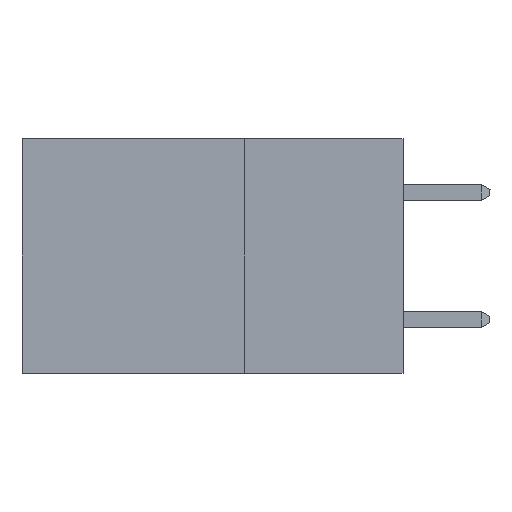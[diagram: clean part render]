
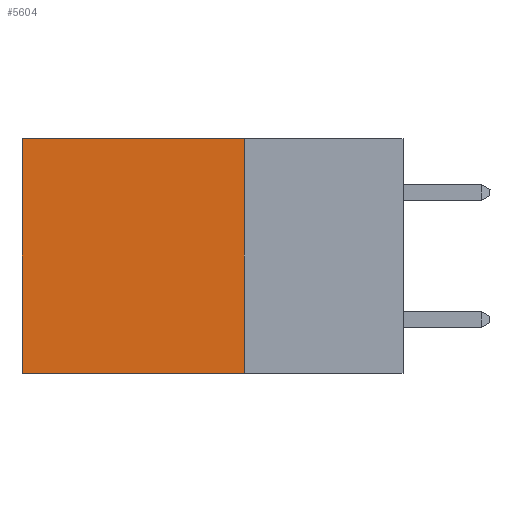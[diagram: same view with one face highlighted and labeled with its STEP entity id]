
A CAD part, left-side view. The second image highlights one B-rep face of the part: STEP entity #5604.
In plain terms, the highlighted planar face has unit normal (-1, 0, 0).
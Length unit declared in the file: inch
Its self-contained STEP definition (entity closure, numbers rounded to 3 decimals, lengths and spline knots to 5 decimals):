
#353 = DIRECTION ( 'NONE',  ( 0., 0., -1. ) ) ;
#376 = CARTESIAN_POINT ( 'NONE',  ( 0.2875, 0.6, 0. ) ) ;
#476 = ORIENTED_EDGE ( 'NONE', *, *, #1804, .F. ) ;
#590 = DIRECTION ( 'NONE',  ( 0., 1., 0. ) ) ;
#1067 = EDGE_CURVE ( 'NONE', #9309, #5365, #3315, .T. ) ;
#1146 = CARTESIAN_POINT ( 'NONE',  ( 0.2875, 0.6, -0.37 ) ) ;
#1309 = ORIENTED_EDGE ( 'NONE', *, *, #3666, .F. ) ;
#1804 = EDGE_CURVE ( 'NONE', #9309, #7388, #7428, .T. ) ;
#2971 = VECTOR ( 'NONE', #5877, 39.37008 ) ;
#3315 = LINE ( 'NONE', #4291, #5368 ) ;
#3666 = EDGE_CURVE ( 'NONE', #7388, #3703, #10018, .T. ) ;
#3703 = VERTEX_POINT ( 'NONE', #1146 ) ;
#3717 = EDGE_CURVE ( 'NONE', #5365, #3703, #4565, .T. ) ;
#3999 = CARTESIAN_POINT ( 'NONE',  ( 0.2875, 0.25, 0. ) ) ;
#4291 = CARTESIAN_POINT ( 'NONE',  ( 0.2875, 0.25, 0. ) ) ;
#4565 = LINE ( 'NONE', #10468, #2971 ) ;
#5197 = CARTESIAN_POINT ( 'NONE',  ( 0.2875, 0.25, -0.37 ) ) ;
#5365 = VERTEX_POINT ( 'NONE', #376 ) ;
#5368 = VECTOR ( 'NONE', #590, 39.37008 ) ;
#5604 = ADVANCED_FACE ( 'NONE', ( #7890 ), #9031, .F. ) ;
#5877 = DIRECTION ( 'NONE',  ( 0., 0., -1. ) ) ;
#6219 = VECTOR ( 'NONE', #11779, 39.37008 ) ;
#6261 = CARTESIAN_POINT ( 'NONE',  ( 0.2875, 0.25, 0. ) ) ;
#6306 = CARTESIAN_POINT ( 'NONE',  ( 0.2875, 0.25, 0. ) ) ;
#7107 = AXIS2_PLACEMENT_3D ( 'NONE', #6306, #10928, #7285 ) ;
#7285 = DIRECTION ( 'NONE',  ( 0., 0., -1. ) ) ;
#7388 = VERTEX_POINT ( 'NONE', #11872 ) ;
#7428 = LINE ( 'NONE', #3999, #10062 ) ;
#7890 = FACE_OUTER_BOUND ( 'NONE', #8282, .T. ) ;
#8010 = ORIENTED_EDGE ( 'NONE', *, *, #3717, .T. ) ;
#8282 = EDGE_LOOP ( 'NONE', ( #8010, #1309, #476, #9195 ) ) ;
#9031 = PLANE ( 'NONE',  #7107 ) ;
#9195 = ORIENTED_EDGE ( 'NONE', *, *, #1067, .T. ) ;
#9309 = VERTEX_POINT ( 'NONE', #6261 ) ;
#10018 = LINE ( 'NONE', #5197, #6219 ) ;
#10062 = VECTOR ( 'NONE', #353, 39.37008 ) ;
#10468 = CARTESIAN_POINT ( 'NONE',  ( 0.2875, 0.6, 0. ) ) ;
#10928 = DIRECTION ( 'NONE',  ( 1., 0., 0. ) ) ;
#11779 = DIRECTION ( 'NONE',  ( 0., 1., 0. ) ) ;
#11872 = CARTESIAN_POINT ( 'NONE',  ( 0.2875, 0.25, -0.37 ) ) ;
